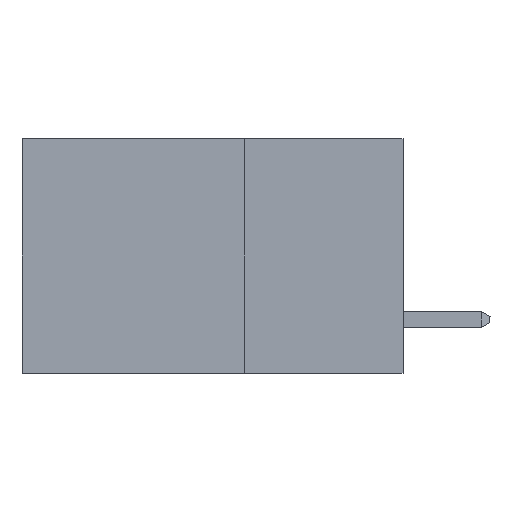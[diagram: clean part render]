
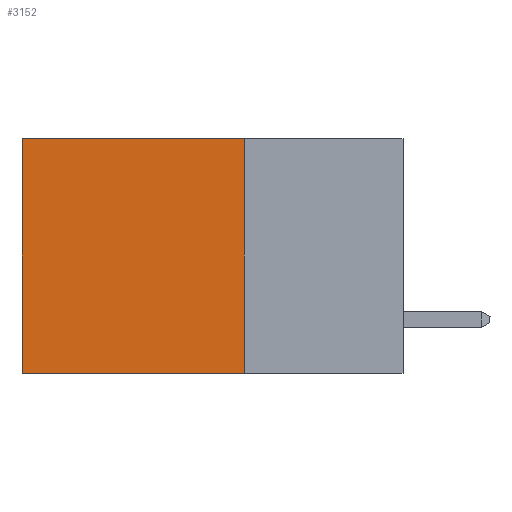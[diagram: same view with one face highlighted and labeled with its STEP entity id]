
A CAD part, left-side view. The second image highlights one B-rep face of the part: STEP entity #3152.
In plain terms, the highlighted planar face has unit normal (-1, 0, 0).
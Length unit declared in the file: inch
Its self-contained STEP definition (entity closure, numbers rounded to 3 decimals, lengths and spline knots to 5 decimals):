
#1749 = DIRECTION ( 'NONE',  ( 0., 1., 0. ) ) ;
#1971 = LINE ( 'NONE', #12597, #7565 ) ;
#3152 = ADVANCED_FACE ( 'NONE', ( #3435 ), #32904, .F. ) ;
#3376 = EDGE_CURVE ( 'NONE', #4840, #18742, #8665, .T. ) ;
#3435 = FACE_OUTER_BOUND ( 'NONE', #22623, .T. ) ;
#4840 = VERTEX_POINT ( 'NONE', #14692 ) ;
#5641 = EDGE_CURVE ( 'NONE', #43959, #27491, #9474, .T. ) ;
#6126 = ORIENTED_EDGE ( 'NONE', *, *, #3376, .T. ) ;
#7394 = EDGE_CURVE ( 'NONE', #4840, #43959, #1971, .T. ) ;
#7565 = VECTOR ( 'NONE', #13525, 39.37008 ) ;
#7969 = CARTESIAN_POINT ( 'NONE',  ( 0.2875, 0.25, 0. ) ) ;
#8355 = ORIENTED_EDGE ( 'NONE', *, *, #5641, .F. ) ;
#8665 = LINE ( 'NONE', #26901, #14660 ) ;
#9474 = LINE ( 'NONE', #41812, #21494 ) ;
#10600 = DIRECTION ( 'NONE',  ( 0., 0., -1. ) ) ;
#12597 = CARTESIAN_POINT ( 'NONE',  ( 0.2875, 0.25, 0. ) ) ;
#13525 = DIRECTION ( 'NONE',  ( 0., 0., -1. ) ) ;
#14660 = VECTOR ( 'NONE', #1749, 39.37008 ) ;
#14692 = CARTESIAN_POINT ( 'NONE',  ( 0.2875, 0.25, 0. ) ) ;
#15666 = CARTESIAN_POINT ( 'NONE',  ( 0.2875, 0.6, 0. ) ) ;
#17322 = LINE ( 'NONE', #31393, #41382 ) ;
#18742 = VERTEX_POINT ( 'NONE', #15666 ) ;
#19836 = AXIS2_PLACEMENT_3D ( 'NONE', #7969, #35070, #10600 ) ;
#19997 = CARTESIAN_POINT ( 'NONE',  ( 0.2875, 0.25, -0.37 ) ) ;
#21494 = VECTOR ( 'NONE', #27029, 39.37008 ) ;
#22623 = EDGE_LOOP ( 'NONE', ( #44930, #8355, #30024, #6126 ) ) ;
#26901 = CARTESIAN_POINT ( 'NONE',  ( 0.2875, 0.25, 0. ) ) ;
#27029 = DIRECTION ( 'NONE',  ( 0., 1., 0. ) ) ;
#27491 = VERTEX_POINT ( 'NONE', #41040 ) ;
#30024 = ORIENTED_EDGE ( 'NONE', *, *, #7394, .F. ) ;
#30061 = EDGE_CURVE ( 'NONE', #18742, #27491, #17322, .T. ) ;
#31393 = CARTESIAN_POINT ( 'NONE',  ( 0.2875, 0.6, 0. ) ) ;
#32904 = PLANE ( 'NONE',  #19836 ) ;
#35070 = DIRECTION ( 'NONE',  ( 1., 0., 0. ) ) ;
#41040 = CARTESIAN_POINT ( 'NONE',  ( 0.2875, 0.6, -0.37 ) ) ;
#41382 = VECTOR ( 'NONE', #45497, 39.37008 ) ;
#41812 = CARTESIAN_POINT ( 'NONE',  ( 0.2875, 0.25, -0.37 ) ) ;
#43959 = VERTEX_POINT ( 'NONE', #19997 ) ;
#44930 = ORIENTED_EDGE ( 'NONE', *, *, #30061, .T. ) ;
#45497 = DIRECTION ( 'NONE',  ( 0., 0., -1. ) ) ;
